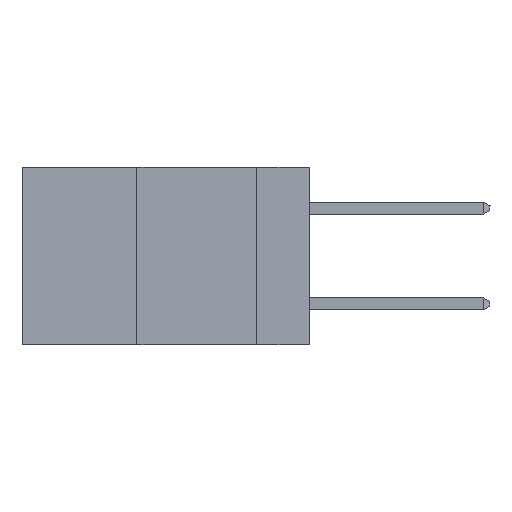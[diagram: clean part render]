
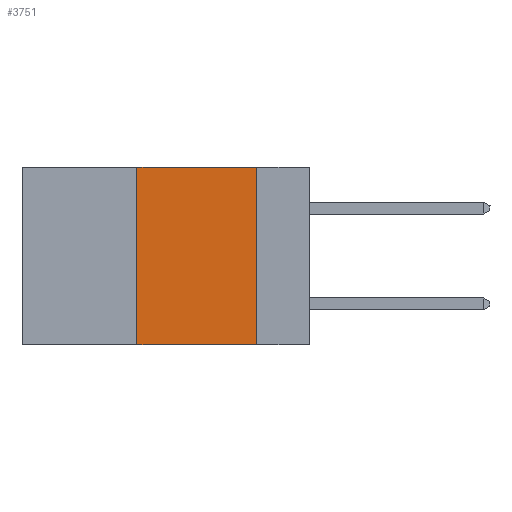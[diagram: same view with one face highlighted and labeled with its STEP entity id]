
A CAD part, left-side view. The second image highlights one B-rep face of the part: STEP entity #3751.
In plain terms, the highlighted planar face has unit normal (-1, 0, 0).
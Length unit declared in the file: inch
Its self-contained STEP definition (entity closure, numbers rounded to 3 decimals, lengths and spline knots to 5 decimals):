
#451 = EDGE_CURVE ( 'NONE', #6864, #4683, #11908, .T. ) ;
#672 = AXIS2_PLACEMENT_3D ( 'NONE', #6653, #9701, #6788 ) ;
#831 = DIRECTION ( 'NONE',  ( 0., 0., -1. ) ) ;
#942 = ORIENTED_EDGE ( 'NONE', *, *, #451, .F. ) ;
#2068 = VERTEX_POINT ( 'NONE', #5362 ) ;
#2115 = DIRECTION ( 'NONE',  ( 0., -1., 0. ) ) ;
#3279 = ORIENTED_EDGE ( 'NONE', *, *, #7191, .F. ) ;
#3634 = ORIENTED_EDGE ( 'NONE', *, *, #11860, .T. ) ;
#3749 = CARTESIAN_POINT ( 'NONE',  ( 0., 0.6, 0. ) ) ;
#3751 = ADVANCED_FACE ( 'NONE', ( #9433 ), #7879, .F. ) ;
#3942 = VERTEX_POINT ( 'NONE', #12126 ) ;
#4112 = CARTESIAN_POINT ( 'NONE',  ( 0., 0.6, -0.37 ) ) ;
#4683 = VERTEX_POINT ( 'NONE', #5331 ) ;
#5161 = VECTOR ( 'NONE', #12032, 39.37008 ) ;
#5331 = CARTESIAN_POINT ( 'NONE',  ( 0., 0.36, 0. ) ) ;
#5362 = CARTESIAN_POINT ( 'NONE',  ( 0., 0.11, -0.37 ) ) ;
#5955 = EDGE_CURVE ( 'NONE', #3942, #2068, #7407, .T. ) ;
#6356 = VECTOR ( 'NONE', #2115, 39.37008 ) ;
#6413 = LINE ( 'NONE', #3749, #7056 ) ;
#6505 = CARTESIAN_POINT ( 'NONE',  ( 0., 0.36, -0.37 ) ) ;
#6653 = CARTESIAN_POINT ( 'NONE',  ( 0., 0.6, 0. ) ) ;
#6741 = DIRECTION ( 'NONE',  ( 0., -1., 0. ) ) ;
#6784 = EDGE_LOOP ( 'NONE', ( #10098, #3279, #942, #3634 ) ) ;
#6788 = DIRECTION ( 'NONE',  ( 0., 0., -1. ) ) ;
#6864 = VERTEX_POINT ( 'NONE', #6505 ) ;
#7056 = VECTOR ( 'NONE', #6741, 39.37008 ) ;
#7191 = EDGE_CURVE ( 'NONE', #4683, #3942, #6413, .T. ) ;
#7407 = LINE ( 'NONE', #11841, #7740 ) ;
#7740 = VECTOR ( 'NONE', #831, 39.37008 ) ;
#7879 = PLANE ( 'NONE',  #672 ) ;
#8895 = CARTESIAN_POINT ( 'NONE',  ( 0., 0.36, 0. ) ) ;
#9433 = FACE_OUTER_BOUND ( 'NONE', #6784, .T. ) ;
#9701 = DIRECTION ( 'NONE',  ( 1., 0., 0. ) ) ;
#10098 = ORIENTED_EDGE ( 'NONE', *, *, #5955, .F. ) ;
#11052 = LINE ( 'NONE', #4112, #6356 ) ;
#11841 = CARTESIAN_POINT ( 'NONE',  ( 0., 0.11, 0. ) ) ;
#11860 = EDGE_CURVE ( 'NONE', #6864, #2068, #11052, .T. ) ;
#11908 = LINE ( 'NONE', #8895, #5161 ) ;
#12032 = DIRECTION ( 'NONE',  ( 0., 0., 1. ) ) ;
#12126 = CARTESIAN_POINT ( 'NONE',  ( 0., 0.11, 0. ) ) ;
